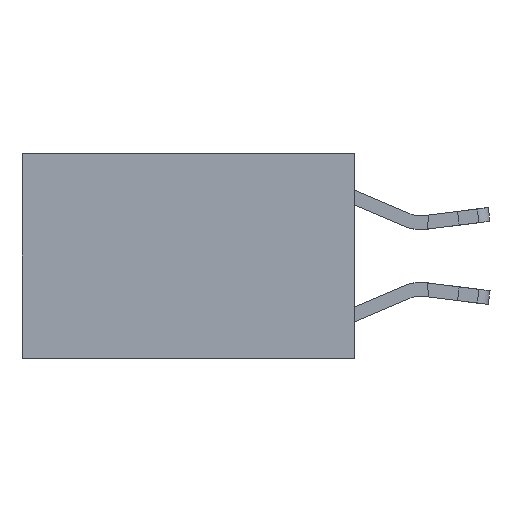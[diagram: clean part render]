
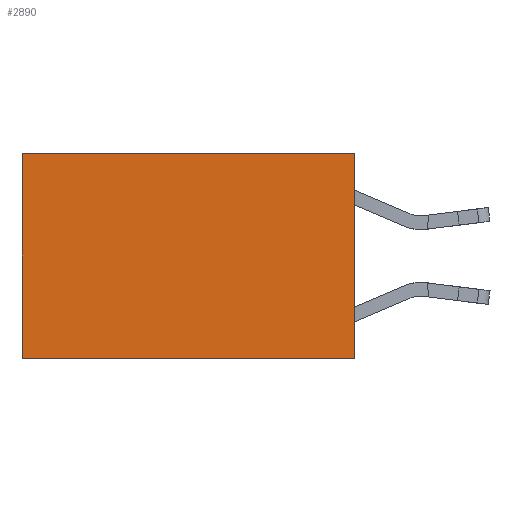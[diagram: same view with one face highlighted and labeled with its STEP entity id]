
A CAD part, left-side view. The second image highlights one B-rep face of the part: STEP entity #2890.
In plain terms, the highlighted planar face has unit normal (-1, 0, 0).
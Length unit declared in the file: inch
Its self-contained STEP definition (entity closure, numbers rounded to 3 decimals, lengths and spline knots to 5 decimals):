
#40 = VERTEX_POINT ( 'NONE', #4127 ) ;
#216 = VERTEX_POINT ( 'NONE', #15125 ) ;
#276 = DIRECTION ( 'NONE',  ( 0., 0., -1. ) ) ;
#1388 = VECTOR ( 'NONE', #2940, 39.37008 ) ;
#1629 = CARTESIAN_POINT ( 'NONE',  ( 0.2625, 0., -0.37 ) ) ;
#2350 = EDGE_LOOP ( 'NONE', ( #2437, #9296, #8906, #2374 ) ) ;
#2374 = ORIENTED_EDGE ( 'NONE', *, *, #13532, .T. ) ;
#2437 = ORIENTED_EDGE ( 'NONE', *, *, #9219, .T. ) ;
#2890 = ADVANCED_FACE ( 'NONE', ( #9697 ), #9269, .F. ) ;
#2940 = DIRECTION ( 'NONE',  ( 0., 1., 0. ) ) ;
#3062 = VERTEX_POINT ( 'NONE', #11775 ) ;
#3126 = CARTESIAN_POINT ( 'NONE',  ( 0.2625, 0., 0. ) ) ;
#3332 = CARTESIAN_POINT ( 'NONE',  ( 0.2625, 0., 0. ) ) ;
#3391 = DIRECTION ( 'NONE',  ( 0., 0., -1. ) ) ;
#4127 = CARTESIAN_POINT ( 'NONE',  ( 0.2625, 0.6, -0.37 ) ) ;
#4891 = CARTESIAN_POINT ( 'NONE',  ( 0.2625, 0., 0. ) ) ;
#5586 = EDGE_CURVE ( 'NONE', #9020, #40, #8244, .T. ) ;
#6701 = CARTESIAN_POINT ( 'NONE',  ( 0.2625, 0.6, 0. ) ) ;
#7541 = LINE ( 'NONE', #6701, #13916 ) ;
#8244 = LINE ( 'NONE', #1629, #1388 ) ;
#8831 = DIRECTION ( 'NONE',  ( 0., 0., -1. ) ) ;
#8906 = ORIENTED_EDGE ( 'NONE', *, *, #14097, .F. ) ;
#8909 = DIRECTION ( 'NONE',  ( 1., 0., 0. ) ) ;
#8966 = LINE ( 'NONE', #3332, #15353 ) ;
#9020 = VERTEX_POINT ( 'NONE', #16474 ) ;
#9219 = EDGE_CURVE ( 'NONE', #216, #40, #7541, .T. ) ;
#9269 = PLANE ( 'NONE',  #11429 ) ;
#9296 = ORIENTED_EDGE ( 'NONE', *, *, #5586, .F. ) ;
#9697 = FACE_OUTER_BOUND ( 'NONE', #2350, .T. ) ;
#10522 = LINE ( 'NONE', #4891, #10932 ) ;
#10932 = VECTOR ( 'NONE', #13803, 39.37008 ) ;
#11429 = AXIS2_PLACEMENT_3D ( 'NONE', #3126, #8909, #8831 ) ;
#11775 = CARTESIAN_POINT ( 'NONE',  ( 0.2625, 0., 0. ) ) ;
#13532 = EDGE_CURVE ( 'NONE', #3062, #216, #10522, .T. ) ;
#13803 = DIRECTION ( 'NONE',  ( 0., 1., 0. ) ) ;
#13916 = VECTOR ( 'NONE', #276, 39.37008 ) ;
#14097 = EDGE_CURVE ( 'NONE', #3062, #9020, #8966, .T. ) ;
#15125 = CARTESIAN_POINT ( 'NONE',  ( 0.2625, 0.6, 0. ) ) ;
#15353 = VECTOR ( 'NONE', #3391, 39.37008 ) ;
#16474 = CARTESIAN_POINT ( 'NONE',  ( 0.2625, 0., -0.37 ) ) ;
